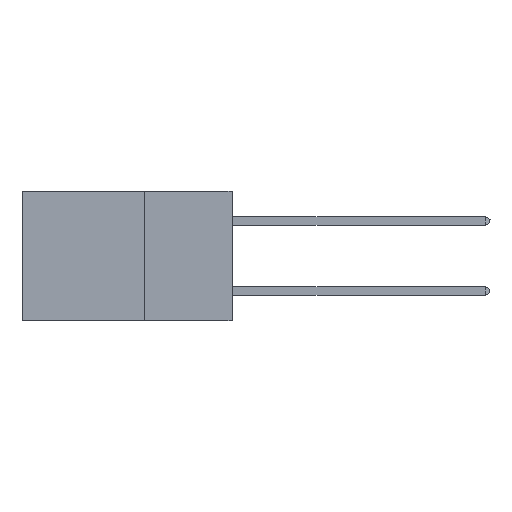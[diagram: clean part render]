
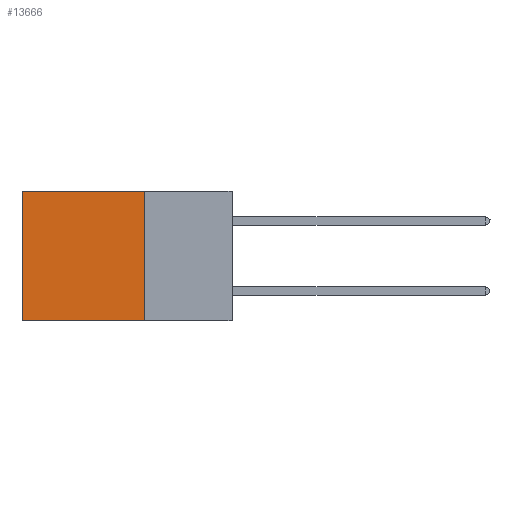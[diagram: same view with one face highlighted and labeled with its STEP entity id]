
A CAD part, left-side view. The second image highlights one B-rep face of the part: STEP entity #13666.
In plain terms, the highlighted planar face has unit normal (-1, 0, 0).
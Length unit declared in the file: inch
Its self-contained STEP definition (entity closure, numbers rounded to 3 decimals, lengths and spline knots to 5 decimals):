
#245 = ORIENTED_EDGE ( 'NONE', *, *, #1400, .F. ) ;
#595 = VECTOR ( 'NONE', #22212, 39.37008 ) ;
#649 = DIRECTION ( 'NONE',  ( 0., 0., -1. ) ) ;
#1240 = ORIENTED_EDGE ( 'NONE', *, *, #10506, .F. ) ;
#1400 = EDGE_CURVE ( 'NONE', #6449, #3034, #18847, .T. ) ;
#1978 = ORIENTED_EDGE ( 'NONE', *, *, #21199, .T. ) ;
#2216 = CARTESIAN_POINT ( 'NONE',  ( 0.2875, 0.25, 0. ) ) ;
#2321 = VERTEX_POINT ( 'NONE', #15725 ) ;
#2511 = CARTESIAN_POINT ( 'NONE',  ( 0.2875, 0.25, -0.37 ) ) ;
#3034 = VERTEX_POINT ( 'NONE', #2511 ) ;
#4456 = CARTESIAN_POINT ( 'NONE',  ( 0.2875, 0.25, 0. ) ) ;
#4541 = DIRECTION ( 'NONE',  ( 0., 1., 0. ) ) ;
#5978 = AXIS2_PLACEMENT_3D ( 'NONE', #22831, #15696, #649 ) ;
#6184 = PLANE ( 'NONE',  #5978 ) ;
#6449 = VERTEX_POINT ( 'NONE', #2216 ) ;
#6469 = DIRECTION ( 'NONE',  ( 0., 1., 0. ) ) ;
#8356 = LINE ( 'NONE', #11869, #21045 ) ;
#8482 = CARTESIAN_POINT ( 'NONE',  ( 0.2875, 0.6, 0. ) ) ;
#9436 = VERTEX_POINT ( 'NONE', #22360 ) ;
#9624 = CARTESIAN_POINT ( 'NONE',  ( 0.2875, 0.25, 0. ) ) ;
#10506 = EDGE_CURVE ( 'NONE', #3034, #9436, #8356, .T. ) ;
#11869 = CARTESIAN_POINT ( 'NONE',  ( 0.2875, 0.25, -0.37 ) ) ;
#13666 = ADVANCED_FACE ( 'NONE', ( #19417 ), #6184, .F. ) ;
#14939 = ORIENTED_EDGE ( 'NONE', *, *, #16174, .T. ) ;
#15696 = DIRECTION ( 'NONE',  ( 1., 0., 0. ) ) ;
#15725 = CARTESIAN_POINT ( 'NONE',  ( 0.2875, 0.6, 0. ) ) ;
#16174 = EDGE_CURVE ( 'NONE', #6449, #2321, #23347, .T. ) ;
#18067 = LINE ( 'NONE', #8482, #21215 ) ;
#18847 = LINE ( 'NONE', #4456, #595 ) ;
#19417 = FACE_OUTER_BOUND ( 'NONE', #22173, .T. ) ;
#21045 = VECTOR ( 'NONE', #4541, 39.37008 ) ;
#21199 = EDGE_CURVE ( 'NONE', #2321, #9436, #18067, .T. ) ;
#21215 = VECTOR ( 'NONE', #21471, 39.37008 ) ;
#21471 = DIRECTION ( 'NONE',  ( 0., 0., -1. ) ) ;
#22173 = EDGE_LOOP ( 'NONE', ( #1978, #1240, #245, #14939 ) ) ;
#22212 = DIRECTION ( 'NONE',  ( 0., 0., -1. ) ) ;
#22360 = CARTESIAN_POINT ( 'NONE',  ( 0.2875, 0.6, -0.37 ) ) ;
#22753 = VECTOR ( 'NONE', #6469, 39.37008 ) ;
#22831 = CARTESIAN_POINT ( 'NONE',  ( 0.2875, 0.25, 0. ) ) ;
#23347 = LINE ( 'NONE', #9624, #22753 ) ;
